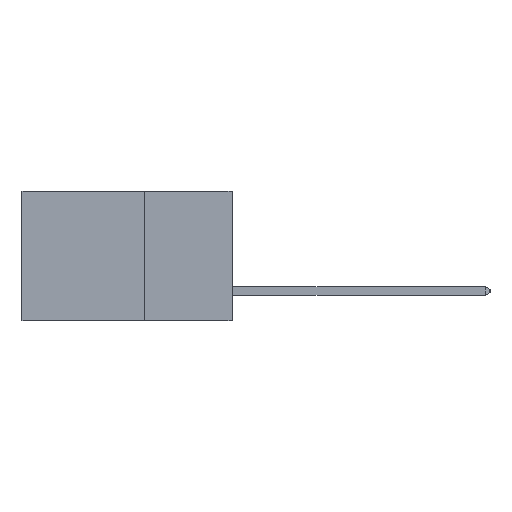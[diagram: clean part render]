
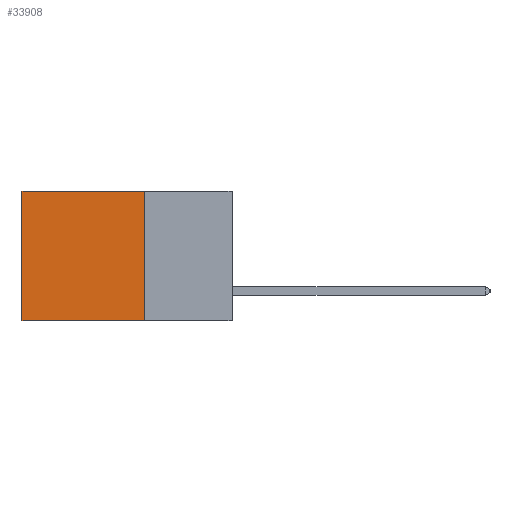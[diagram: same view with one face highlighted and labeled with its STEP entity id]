
A CAD part, left-side view. The second image highlights one B-rep face of the part: STEP entity #33908.
In plain terms, the highlighted planar face has unit normal (-1, 0, 0).
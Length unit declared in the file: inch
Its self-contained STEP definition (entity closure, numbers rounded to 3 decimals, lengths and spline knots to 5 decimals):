
#310 = VERTEX_POINT ( 'NONE', #31035 ) ;
#1089 = CARTESIAN_POINT ( 'NONE',  ( 0.2875, 0.25, -0.37 ) ) ;
#4176 = DIRECTION ( 'NONE',  ( 0., 1., 0. ) ) ;
#6134 = DIRECTION ( 'NONE',  ( 0., 0., -1. ) ) ;
#6809 = CARTESIAN_POINT ( 'NONE',  ( 0.2875, 0.6, -0.37 ) ) ;
#7919 = VERTEX_POINT ( 'NONE', #24773 ) ;
#9088 = EDGE_CURVE ( 'NONE', #310, #28428, #19450, .T. ) ;
#11365 = VECTOR ( 'NONE', #12829, 39.37008 ) ;
#11699 = VECTOR ( 'NONE', #28315, 39.37008 ) ;
#12829 = DIRECTION ( 'NONE',  ( 0., 1., 0. ) ) ;
#14711 = ORIENTED_EDGE ( 'NONE', *, *, #36223, .T. ) ;
#14998 = EDGE_CURVE ( 'NONE', #310, #7919, #27587, .T. ) ;
#15687 = DIRECTION ( 'NONE',  ( 0., 0., -1. ) ) ;
#16417 = CARTESIAN_POINT ( 'NONE',  ( 0.2875, 0.6, 0. ) ) ;
#16861 = PLANE ( 'NONE',  #29959 ) ;
#18743 = CARTESIAN_POINT ( 'NONE',  ( 0.2875, 0.25, 0. ) ) ;
#19450 = LINE ( 'NONE', #30970, #11365 ) ;
#21230 = CARTESIAN_POINT ( 'NONE',  ( 0.2875, 0.25, 0. ) ) ;
#21632 = LINE ( 'NONE', #1089, #36561 ) ;
#23246 = EDGE_LOOP ( 'NONE', ( #14711, #25032, #28914, #35466 ) ) ;
#24223 = DIRECTION ( 'NONE',  ( 1., 0., 0. ) ) ;
#24773 = CARTESIAN_POINT ( 'NONE',  ( 0.2875, 0.25, -0.37 ) ) ;
#25032 = ORIENTED_EDGE ( 'NONE', *, *, #36219, .F. ) ;
#25314 = CARTESIAN_POINT ( 'NONE',  ( 0.2875, 0.6, 0. ) ) ;
#27587 = LINE ( 'NONE', #18743, #34587 ) ;
#27712 = LINE ( 'NONE', #25314, #11699 ) ;
#28315 = DIRECTION ( 'NONE',  ( 0., 0., -1. ) ) ;
#28428 = VERTEX_POINT ( 'NONE', #16417 ) ;
#28914 = ORIENTED_EDGE ( 'NONE', *, *, #14998, .F. ) ;
#29959 = AXIS2_PLACEMENT_3D ( 'NONE', #21230, #24223, #6134 ) ;
#30970 = CARTESIAN_POINT ( 'NONE',  ( 0.2875, 0.25, 0. ) ) ;
#31035 = CARTESIAN_POINT ( 'NONE',  ( 0.2875, 0.25, 0. ) ) ;
#33908 = ADVANCED_FACE ( 'NONE', ( #38163 ), #16861, .F. ) ;
#34587 = VECTOR ( 'NONE', #15687, 39.37008 ) ;
#35466 = ORIENTED_EDGE ( 'NONE', *, *, #9088, .T. ) ;
#36219 = EDGE_CURVE ( 'NONE', #7919, #38553, #21632, .T. ) ;
#36223 = EDGE_CURVE ( 'NONE', #28428, #38553, #27712, .T. ) ;
#36561 = VECTOR ( 'NONE', #4176, 39.37008 ) ;
#38163 = FACE_OUTER_BOUND ( 'NONE', #23246, .T. ) ;
#38553 = VERTEX_POINT ( 'NONE', #6809 ) ;
